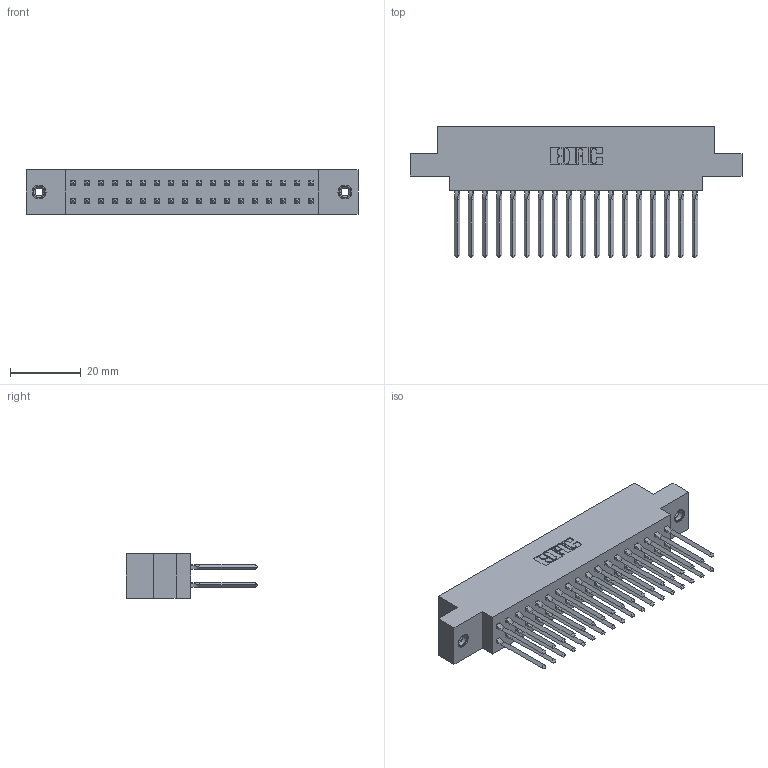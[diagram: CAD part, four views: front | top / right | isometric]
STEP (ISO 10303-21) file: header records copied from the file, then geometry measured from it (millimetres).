
FILE_DESCRIPTION (( 'STEP AP203' ), '1' );
FILE_NAME ('317-036-540-878.STEP', '2020-02-27T22:48:43', ( '' ), ( '' ), 'SwSTEP 2.0', 'SolidWorks 2016', '' );
FILE_SCHEMA (( 'CONFIG_CONTROL_DESIGN' ));
Length unit declared in the file: inch
Products named in the file (4): 317 Part_.156 Dia - TI; 345-250-001_345-250-003-102; 317-290-001_540; 317-036-540-878
Assembly tree (39 placements, depth 2):
  317-036-540-878
    317 Part_.156 Dia - TI
    317-290-001_540  x36
    345-250-001_345-250-003-102  x2
Bounding box: 94.03 x 37.34 x 12.7 mm (x, y, z)
Volume: 14963.3 mm3; surface area: 21424.6 mm2
Topology: 39 solids, 39 shells, 3366 faces, 9303 edges, 5990 vertices
Faces by surface type: plane 2718, cylinder 488, bspline 144, cone 12, torus 4
Entity records: 30553 total; most frequent: CARTESIAN_POINT 5714, ORIENTED_EDGE 5206, DIRECTION 4387, EDGE_CURVE 2603, VECTOR 2327, LINE 2327, VERTEX_POINT 1725, AXIS2_PLACEMENT_3D 1030
